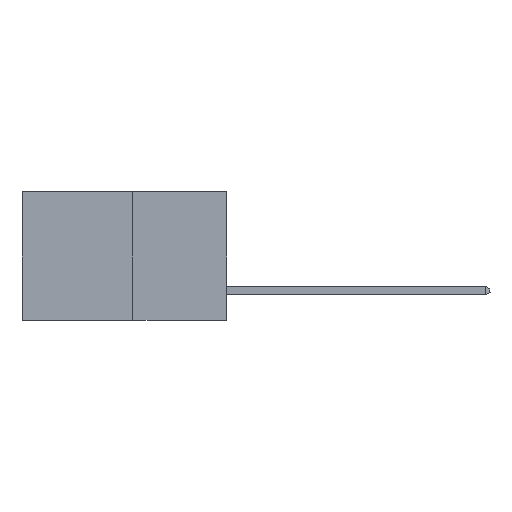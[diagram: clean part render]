
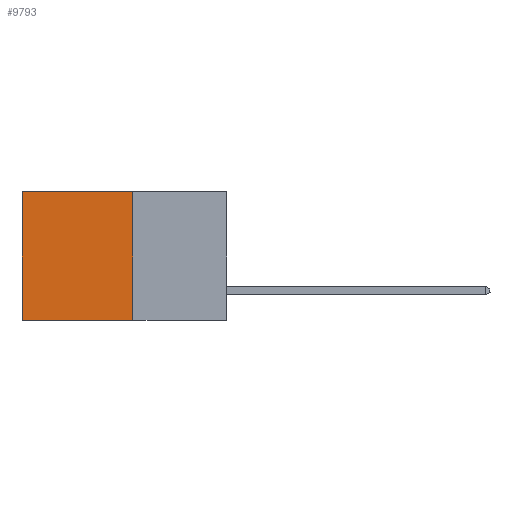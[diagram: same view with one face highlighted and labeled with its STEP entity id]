
A CAD part, left-side view. The second image highlights one B-rep face of the part: STEP entity #9793.
In plain terms, the highlighted planar face has unit normal (-1, 0, 0).
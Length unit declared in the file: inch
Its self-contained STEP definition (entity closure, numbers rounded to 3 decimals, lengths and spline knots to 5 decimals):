
#208 = CARTESIAN_POINT ( 'NONE',  ( 0.277, 0.27, 0. ) ) ;
#817 = VERTEX_POINT ( 'NONE', #7836 ) ;
#1161 = PLANE ( 'NONE',  #1520 ) ;
#1466 = CARTESIAN_POINT ( 'NONE',  ( 0.277, 0.27, -0.37 ) ) ;
#1520 = AXIS2_PLACEMENT_3D ( 'NONE', #2536, #10388, #3794 ) ;
#2484 = FACE_OUTER_BOUND ( 'NONE', #13281, .T. ) ;
#2536 = CARTESIAN_POINT ( 'NONE',  ( 0.277, 0.27, -0.37 ) ) ;
#2796 = LINE ( 'NONE', #208, #5526 ) ;
#3794 = DIRECTION ( 'NONE',  ( 0., 0., -1. ) ) ;
#3910 = VERTEX_POINT ( 'NONE', #4190 ) ;
#4190 = CARTESIAN_POINT ( 'NONE',  ( 0.277, 0.59, -0.37 ) ) ;
#4441 = EDGE_CURVE ( 'NONE', #817, #3910, #10527, .T. ) ;
#4587 = CARTESIAN_POINT ( 'NONE',  ( 0.277, 0.59, -0.37 ) ) ;
#4869 = DIRECTION ( 'NONE',  ( 0., 0., -1. ) ) ;
#5185 = DIRECTION ( 'NONE',  ( 0., 1., 0. ) ) ;
#5210 = CARTESIAN_POINT ( 'NONE',  ( 0.277, 0.59, 0. ) ) ;
#5510 = LINE ( 'NONE', #12412, #11263 ) ;
#5526 = VECTOR ( 'NONE', #10711, 39.37008 ) ;
#7309 = EDGE_CURVE ( 'NONE', #8800, #10907, #2796, .T. ) ;
#7836 = CARTESIAN_POINT ( 'NONE',  ( 0.277, 0.27, -0.37 ) ) ;
#7963 = DIRECTION ( 'NONE',  ( 0., 0., -1. ) ) ;
#7970 = EDGE_CURVE ( 'NONE', #8800, #817, #5510, .T. ) ;
#8800 = VERTEX_POINT ( 'NONE', #10402 ) ;
#9111 = VECTOR ( 'NONE', #7963, 39.37008 ) ;
#9233 = ORIENTED_EDGE ( 'NONE', *, *, #9324, .T. ) ;
#9324 = EDGE_CURVE ( 'NONE', #10907, #3910, #12173, .T. ) ;
#9372 = ORIENTED_EDGE ( 'NONE', *, *, #7970, .F. ) ;
#9793 = ADVANCED_FACE ( 'NONE', ( #2484 ), #1161, .F. ) ;
#10388 = DIRECTION ( 'NONE',  ( 1., 0., 0. ) ) ;
#10402 = CARTESIAN_POINT ( 'NONE',  ( 0.277, 0.27, 0. ) ) ;
#10527 = LINE ( 'NONE', #1466, #12925 ) ;
#10711 = DIRECTION ( 'NONE',  ( 0., 1., 0. ) ) ;
#10774 = ORIENTED_EDGE ( 'NONE', *, *, #4441, .F. ) ;
#10907 = VERTEX_POINT ( 'NONE', #5210 ) ;
#11263 = VECTOR ( 'NONE', #4869, 39.37008 ) ;
#12173 = LINE ( 'NONE', #4587, #9111 ) ;
#12412 = CARTESIAN_POINT ( 'NONE',  ( 0.277, 0.27, -0.37 ) ) ;
#12925 = VECTOR ( 'NONE', #5185, 39.37008 ) ;
#13281 = EDGE_LOOP ( 'NONE', ( #9233, #10774, #9372, #13655 ) ) ;
#13655 = ORIENTED_EDGE ( 'NONE', *, *, #7309, .T. ) ;
